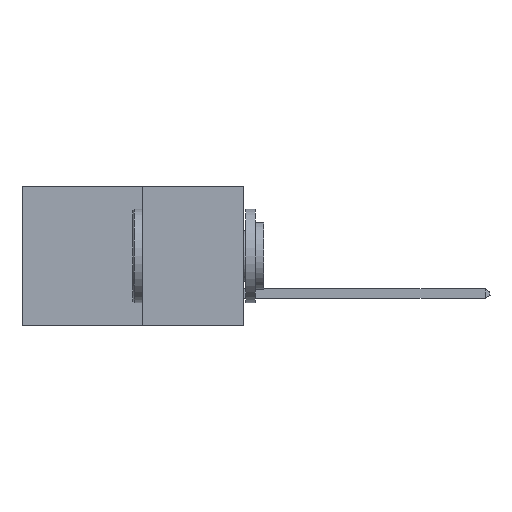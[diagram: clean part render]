
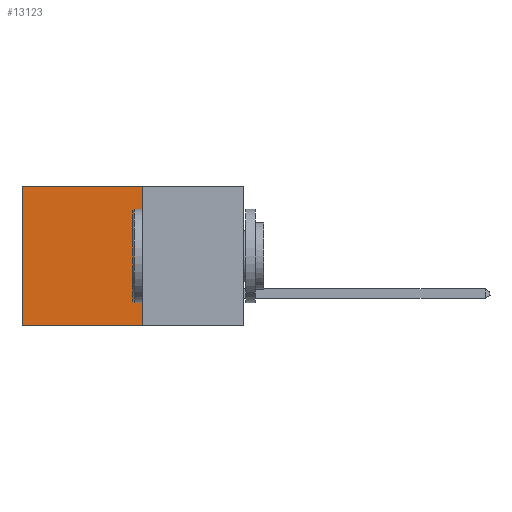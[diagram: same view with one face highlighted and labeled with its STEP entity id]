
A CAD part, left-side view. The second image highlights one B-rep face of the part: STEP entity #13123.
In plain terms, the highlighted planar face has unit normal (-1, 0, 0).
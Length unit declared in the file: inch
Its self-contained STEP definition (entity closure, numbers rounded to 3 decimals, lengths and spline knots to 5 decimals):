
#1479 = LINE ( 'NONE', #11093, #10340 ) ;
#1930 = CARTESIAN_POINT ( 'NONE',  ( 0.277, 0.27, -0.37 ) ) ;
#2123 = CARTESIAN_POINT ( 'NONE',  ( 0.277, 0.59, -0.37 ) ) ;
#2326 = CARTESIAN_POINT ( 'NONE',  ( 0.277, 0.59, -0.37 ) ) ;
#2885 = CARTESIAN_POINT ( 'NONE',  ( 0.277, 0.27, -0.37 ) ) ;
#3829 = FACE_OUTER_BOUND ( 'NONE', #12536, .T. ) ;
#3953 = LINE ( 'NONE', #11425, #10310 ) ;
#4358 = DIRECTION ( 'NONE',  ( 0., 0., -1. ) ) ;
#4566 = EDGE_CURVE ( 'NONE', #6666, #9317, #1479, .T. ) ;
#5146 = CARTESIAN_POINT ( 'NONE',  ( 0.277, 0.59, 0. ) ) ;
#5698 = LINE ( 'NONE', #2326, #14729 ) ;
#5816 = DIRECTION ( 'NONE',  ( 0., 0., -1. ) ) ;
#5833 = AXIS2_PLACEMENT_3D ( 'NONE', #11684, #12753, #5816 ) ;
#6666 = VERTEX_POINT ( 'NONE', #10992 ) ;
#6913 = VERTEX_POINT ( 'NONE', #2885 ) ;
#8748 = ORIENTED_EDGE ( 'NONE', *, *, #4566, .T. ) ;
#8908 = VERTEX_POINT ( 'NONE', #2123 ) ;
#9187 = ORIENTED_EDGE ( 'NONE', *, *, #11860, .F. ) ;
#9317 = VERTEX_POINT ( 'NONE', #5146 ) ;
#9430 = PLANE ( 'NONE',  #5833 ) ;
#9436 = ORIENTED_EDGE ( 'NONE', *, *, #10997, .T. ) ;
#10310 = VECTOR ( 'NONE', #4358, 39.37008 ) ;
#10340 = VECTOR ( 'NONE', #11265, 39.37008 ) ;
#10692 = DIRECTION ( 'NONE',  ( 0., 0., -1. ) ) ;
#10992 = CARTESIAN_POINT ( 'NONE',  ( 0.277, 0.27, 0. ) ) ;
#10997 = EDGE_CURVE ( 'NONE', #9317, #8908, #5698, .T. ) ;
#11093 = CARTESIAN_POINT ( 'NONE',  ( 0.277, 0.27, 0. ) ) ;
#11265 = DIRECTION ( 'NONE',  ( 0., 1., 0. ) ) ;
#11425 = CARTESIAN_POINT ( 'NONE',  ( 0.277, 0.27, -0.37 ) ) ;
#11447 = DIRECTION ( 'NONE',  ( 0., 1., 0. ) ) ;
#11684 = CARTESIAN_POINT ( 'NONE',  ( 0.277, 0.27, -0.37 ) ) ;
#11860 = EDGE_CURVE ( 'NONE', #6913, #8908, #14707, .T. ) ;
#12536 = EDGE_LOOP ( 'NONE', ( #9436, #9187, #14331, #8748 ) ) ;
#12753 = DIRECTION ( 'NONE',  ( 1., 0., 0. ) ) ;
#13123 = ADVANCED_FACE ( 'NONE', ( #3829 ), #9430, .F. ) ;
#14331 = ORIENTED_EDGE ( 'NONE', *, *, #14456, .F. ) ;
#14380 = VECTOR ( 'NONE', #11447, 39.37008 ) ;
#14456 = EDGE_CURVE ( 'NONE', #6666, #6913, #3953, .T. ) ;
#14707 = LINE ( 'NONE', #1930, #14380 ) ;
#14729 = VECTOR ( 'NONE', #10692, 39.37008 ) ;
